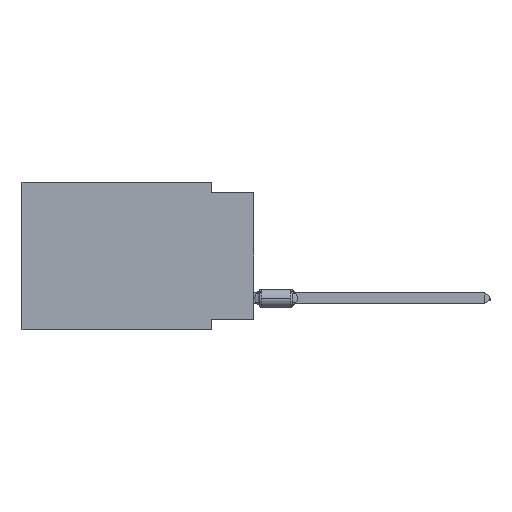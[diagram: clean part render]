
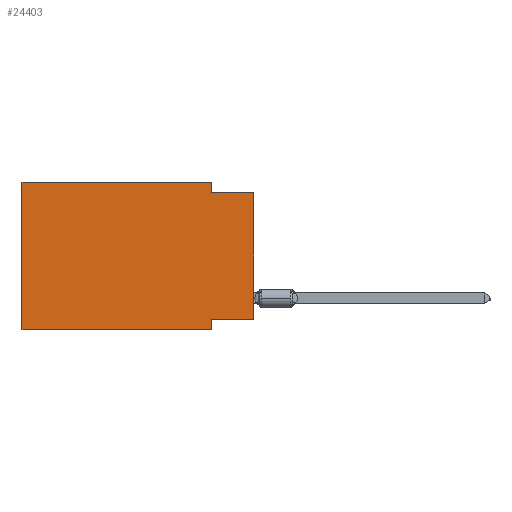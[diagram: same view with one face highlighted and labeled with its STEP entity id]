
A CAD part, left-side view. The second image highlights one B-rep face of the part: STEP entity #24403.
In plain terms, the highlighted planar face has unit normal (-1, 0, 0).
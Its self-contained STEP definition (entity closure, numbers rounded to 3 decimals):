
#463 = CARTESIAN_POINT ( 'NONE',  ( 0., 13.97, 0. ) ) ;
#914 = VERTEX_POINT ( 'NONE', #28959 ) ;
#1049 = VECTOR ( 'NONE', #11751, 1000. ) ;
#1191 = EDGE_CURVE ( 'NONE', #14431, #21872, #2030, .T. ) ;
#1741 = VECTOR ( 'NONE', #17196, 1000. ) ;
#2030 = LINE ( 'NONE', #11522, #12309 ) ;
#2120 = VECTOR ( 'NONE', #29461, 1000. ) ;
#3008 = FACE_OUTER_BOUND ( 'NONE', #15467, .T. ) ;
#3896 = VERTEX_POINT ( 'NONE', #6711 ) ;
#4863 = DIRECTION ( 'NONE',  ( 1., 0., 0. ) ) ;
#5395 = DIRECTION ( 'NONE',  ( 0., 1., 0. ) ) ;
#5893 = CARTESIAN_POINT ( 'NONE',  ( 0., 13.97, 0. ) ) ;
#6711 = CARTESIAN_POINT ( 'NONE',  ( 0., 0., -0.635 ) ) ;
#6790 = CARTESIAN_POINT ( 'NONE',  ( 0., 2.54, 0. ) ) ;
#7567 = VERTEX_POINT ( 'NONE', #9817 ) ;
#7585 = ORIENTED_EDGE ( 'NONE', *, *, #13740, .T. ) ;
#7813 = CARTESIAN_POINT ( 'NONE',  ( 0., 2.54, -8.89 ) ) ;
#9817 = CARTESIAN_POINT ( 'NONE',  ( 0., 2.54, -8.89 ) ) ;
#10142 = CARTESIAN_POINT ( 'NONE',  ( 0., 0., -8.255 ) ) ;
#10411 = AXIS2_PLACEMENT_3D ( 'NONE', #24090, #4863, #23788 ) ;
#10980 = EDGE_CURVE ( 'NONE', #914, #20769, #22004, .T. ) ;
#11522 = CARTESIAN_POINT ( 'NONE',  ( 0., 2.54, 0. ) ) ;
#11751 = DIRECTION ( 'NONE',  ( 0., -1., 0. ) ) ;
#12309 = VECTOR ( 'NONE', #30046, 1000. ) ;
#13740 = EDGE_CURVE ( 'NONE', #914, #7567, #15948, .T. ) ;
#13919 = CARTESIAN_POINT ( 'NONE',  ( 0., 13.97, -8.89 ) ) ;
#14076 = PLANE ( 'NONE',  #10411 ) ;
#14431 = VERTEX_POINT ( 'NONE', #6790 ) ;
#14575 = CARTESIAN_POINT ( 'NONE',  ( 0., 2.54, -8.255 ) ) ;
#15467 = EDGE_LOOP ( 'NONE', ( #28953, #30040, #30427, #18917, #21588, #7585, #16083, #21683 ) ) ;
#15691 = DIRECTION ( 'NONE',  ( 0., -1., 0. ) ) ;
#15761 = DIRECTION ( 'NONE',  ( 0., 0., 1. ) ) ;
#15948 = LINE ( 'NONE', #13919, #1049 ) ;
#16083 = ORIENTED_EDGE ( 'NONE', *, *, #28356, .F. ) ;
#16602 = VERTEX_POINT ( 'NONE', #28677 ) ;
#17065 = DIRECTION ( 'NONE',  ( 0., 0., 1. ) ) ;
#17196 = DIRECTION ( 'NONE',  ( 0., 0., -1. ) ) ;
#17388 = CARTESIAN_POINT ( 'NONE',  ( 0., 13.97, 0. ) ) ;
#17772 = EDGE_CURVE ( 'NONE', #16602, #3896, #27646, .T. ) ;
#18387 = CARTESIAN_POINT ( 'NONE',  ( 0., 0., 0. ) ) ;
#18917 = ORIENTED_EDGE ( 'NONE', *, *, #24977, .F. ) ;
#19519 = LINE ( 'NONE', #7813, #1741 ) ;
#19563 = VECTOR ( 'NONE', #15691, 1000. ) ;
#19661 = VECTOR ( 'NONE', #17065, 1000. ) ;
#20320 = CARTESIAN_POINT ( 'NONE',  ( 0., 0., -0.635 ) ) ;
#20769 = VERTEX_POINT ( 'NONE', #17388 ) ;
#20838 = EDGE_CURVE ( 'NONE', #16602, #21192, #29276, .T. ) ;
#21192 = VERTEX_POINT ( 'NONE', #14575 ) ;
#21472 = VECTOR ( 'NONE', #5395, 1000. ) ;
#21588 = ORIENTED_EDGE ( 'NONE', *, *, #10980, .F. ) ;
#21683 = ORIENTED_EDGE ( 'NONE', *, *, #20838, .F. ) ;
#21872 = VERTEX_POINT ( 'NONE', #29925 ) ;
#22004 = LINE ( 'NONE', #463, #19661 ) ;
#22257 = EDGE_CURVE ( 'NONE', #21872, #3896, #22481, .T. ) ;
#22481 = LINE ( 'NONE', #20320, #19563 ) ;
#23788 = DIRECTION ( 'NONE',  ( 0., 0., -1. ) ) ;
#24090 = CARTESIAN_POINT ( 'NONE',  ( 0., 13.97, 0. ) ) ;
#24203 = LINE ( 'NONE', #5893, #2120 ) ;
#24403 = ADVANCED_FACE ( 'NONE', ( #3008 ), #14076, .F. ) ;
#24815 = VECTOR ( 'NONE', #15761, 1000. ) ;
#24977 = EDGE_CURVE ( 'NONE', #20769, #14431, #24203, .T. ) ;
#27646 = LINE ( 'NONE', #18387, #24815 ) ;
#28356 = EDGE_CURVE ( 'NONE', #21192, #7567, #19519, .T. ) ;
#28677 = CARTESIAN_POINT ( 'NONE',  ( 0., 0., -8.255 ) ) ;
#28953 = ORIENTED_EDGE ( 'NONE', *, *, #17772, .T. ) ;
#28959 = CARTESIAN_POINT ( 'NONE',  ( 0., 13.97, -8.89 ) ) ;
#29276 = LINE ( 'NONE', #10142, #21472 ) ;
#29461 = DIRECTION ( 'NONE',  ( 0., -1., 0. ) ) ;
#29925 = CARTESIAN_POINT ( 'NONE',  ( 0., 2.54, -0.635 ) ) ;
#30040 = ORIENTED_EDGE ( 'NONE', *, *, #22257, .F. ) ;
#30046 = DIRECTION ( 'NONE',  ( 0., 0., -1. ) ) ;
#30427 = ORIENTED_EDGE ( 'NONE', *, *, #1191, .F. ) ;
